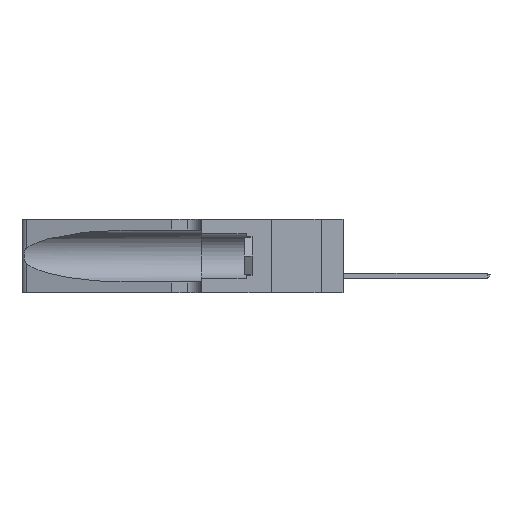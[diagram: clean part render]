
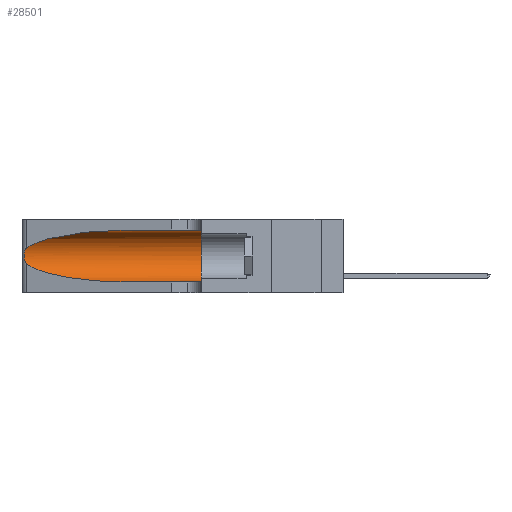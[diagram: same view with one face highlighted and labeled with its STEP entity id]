
A CAD part, left-side view. The second image highlights one B-rep face of the part: STEP entity #28501.
In plain terms, the highlighted cylindrical face has radius 3.308 mm (diameter 6.617 mm), a partial arc.
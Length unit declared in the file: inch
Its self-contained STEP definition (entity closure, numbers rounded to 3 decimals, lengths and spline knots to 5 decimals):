
#901 = VECTOR ( 'NONE', #15719, 39.37008 ) ;
#1679 = DIRECTION ( 'NONE',  ( 0., -1., 0. ) ) ;
#1787 = CARTESIAN_POINT ( 'NONE',  ( 0.1305, 0.72297, 0.31525 ) ) ;
#2654 = CARTESIAN_POINT ( 'NONE',  ( 0.25487, 1.22718, 0.14631 ) ) ;
#3129 = CARTESIAN_POINT ( 'NONE',  ( 0.25487, 1.22718, 0.22369 ) ) ;
#4407 = ORIENTED_EDGE ( 'NONE', *, *, #14760, .F. ) ;
#6469 = EDGE_CURVE ( 'NONE', #27882, #23097, #34751, .T. ) ;
#7777 = CARTESIAN_POINT ( 'NONE',  ( 0.25789, 1.23486, 0.15765 ) ) ;
#8193 = CARTESIAN_POINT ( 'NONE',  ( 0.2373, 1.15595, 0.28018 ) ) ;
#9518 = AXIS2_PLACEMENT_3D ( 'NONE', #21501, #12907, #29490 ) ;
#10396 = DIRECTION ( 'NONE',  ( 0., 0., 1. ) ) ;
#10615 = DIRECTION ( 'NONE',  ( 0., 1., 0. ) ) ;
#10787 = ORIENTED_EDGE ( 'NONE', *, *, #6469, .T. ) ;
#11015 = CARTESIAN_POINT ( 'NONE',  ( 0.1305, 0.72297, 0.31525 ) ) ;
#11675 = CARTESIAN_POINT ( 'NONE',  ( 0.1305, 0.72297, 0.05475 ) ) ;
#12907 = DIRECTION ( 'NONE',  ( 0., -1., 0. ) ) ;
#13051 = EDGE_CURVE ( 'NONE', #18614, #27882, #20097, .T. ) ;
#13065 = EDGE_LOOP ( 'NONE', ( #19049, #10787, #21907, #31096, #4407, #27449 ) ) ;
#13212 = CARTESIAN_POINT ( 'NONE',  ( 0.25639, 1.23186, 0.15144 ) ) ;
#13287 = CARTESIAN_POINT ( 'NONE',  ( 0.25787, 1.23484, 0.2124 ) ) ;
#14752 = CARTESIAN_POINT ( 'NONE',  ( 0.26017, 1.23833, 0.17102 ) ) ;
#14760 = EDGE_CURVE ( 'NONE', #23066, #15373, #33604, .T. ) ;
#15373 = VERTEX_POINT ( 'NONE', #18941 ) ;
#15399 = LINE ( 'NONE', #28543, #28885 ) ;
#15586 = CARTESIAN_POINT ( 'NONE',  ( 0.1305, 1.61858, 0.05475 ) ) ;
#15719 = DIRECTION ( 'NONE',  ( 0., -1., 0. ) ) ;
#16036 = FACE_OUTER_BOUND ( 'NONE', #13065, .T. ) ;
#16269 = CARTESIAN_POINT ( 'NONE',  ( 0.25487, 1.22718, 0.22369 ) ) ;
#17012 = AXIS2_PLACEMENT_3D ( 'NONE', #31837, #10615, #10396 ) ;
#17485 = CARTESIAN_POINT ( 'NONE',  ( 0.25639, 1.23184, 0.21858 ) ) ;
#18572 = CARTESIAN_POINT ( 'NONE',  ( 0.1305, 0.72297, 0.05475 ) ) ;
#18614 = VERTEX_POINT ( 'NONE', #1787 ) ;
#18941 = CARTESIAN_POINT ( 'NONE',  ( 0.1305, 0.35, 0.05475 ) ) ;
#18957 = CARTESIAN_POINT ( 'NONE',  ( 0.25555, 1.22993, 0.14849 ) ) ;
#19049 = ORIENTED_EDGE ( 'NONE', *, *, #13051, .T. ) ;
#19261 = CARTESIAN_POINT ( 'NONE',  ( 0.18966, 0.96281, 0.31525 ) ) ;
#20068 = EDGE_CURVE ( 'NONE', #23097, #29409, #21814, .T. ) ;
#20097 =( BOUNDED_CURVE ( )  B_SPLINE_CURVE ( 3, ( #11015, #19261, #8193, #3129 ),
 .UNSPECIFIED., .F., .F. ) 
 B_SPLINE_CURVE_WITH_KNOTS ( ( 4, 4 ),
 ( 1.5708, 2.84003 ),
 .UNSPECIFIED. ) 
 CURVE ( )  GEOMETRIC_REPRESENTATION_ITEM ( )  RATIONAL_B_SPLINE_CURVE ( ( 1., 0.87, 0.87, 1. ) ) 
 REPRESENTATION_ITEM ( '' )  );
#21279 = CARTESIAN_POINT ( 'NONE',  ( 0.25854, 1.2359, 0.20912 ) ) ;
#21501 = CARTESIAN_POINT ( 'NONE',  ( 0.1305, 1.61858, 0.185 ) ) ;
#21814 =( BOUNDED_CURVE ( )  B_SPLINE_CURVE ( 3, ( #2654, #29160, #25000, #11675 ),
 .UNSPECIFIED., .F., .F. ) 
 B_SPLINE_CURVE_WITH_KNOTS ( ( 4, 4 ),
 ( 3.44316, 4.71239 ),
 .UNSPECIFIED. ) 
 CURVE ( )  GEOMETRIC_REPRESENTATION_ITEM ( )  RATIONAL_B_SPLINE_CURVE ( ( 1., 0.87, 0.87, 1. ) ) 
 REPRESENTATION_ITEM ( '' )  );
#21907 = ORIENTED_EDGE ( 'NONE', *, *, #20068, .T. ) ;
#22245 = EDGE_CURVE ( 'NONE', #29409, #15373, #26633, .T. ) ;
#22837 = CARTESIAN_POINT ( 'NONE',  ( 0.26075, 1.23896, 0.178 ) ) ;
#23066 = VERTEX_POINT ( 'NONE', #32313 ) ;
#23097 = VERTEX_POINT ( 'NONE', #24535 ) ;
#24397 = CARTESIAN_POINT ( 'NONE',  ( 0.25487, 1.22718, 0.14631 ) ) ;
#24535 = CARTESIAN_POINT ( 'NONE',  ( 0.25487, 1.22718, 0.14631 ) ) ;
#25000 = CARTESIAN_POINT ( 'NONE',  ( 0.18966, 0.96281, 0.05475 ) ) ;
#26152 = CARTESIAN_POINT ( 'NONE',  ( 0.26018, 1.23835, 0.19895 ) ) ;
#26425 = EDGE_CURVE ( 'NONE', #18614, #23066, #15399, .T. ) ;
#26633 = LINE ( 'NONE', #15586, #901 ) ;
#27449 = ORIENTED_EDGE ( 'NONE', *, *, #26425, .F. ) ;
#27882 = VERTEX_POINT ( 'NONE', #29416 ) ;
#28501 = ADVANCED_FACE ( 'NONE', ( #16036 ), #33329, .F. ) ;
#28543 = CARTESIAN_POINT ( 'NONE',  ( 0.1305, 1.61858, 0.31525 ) ) ;
#28885 = VECTOR ( 'NONE', #1679, 39.37008 ) ;
#29160 = CARTESIAN_POINT ( 'NONE',  ( 0.2373, 1.15595, 0.08982 ) ) ;
#29409 = VERTEX_POINT ( 'NONE', #18572 ) ;
#29416 = CARTESIAN_POINT ( 'NONE',  ( 0.25487, 1.22718, 0.22369 ) ) ;
#29490 = DIRECTION ( 'NONE',  ( 0., 0., -1. ) ) ;
#31096 = ORIENTED_EDGE ( 'NONE', *, *, #22245, .T. ) ;
#31837 = CARTESIAN_POINT ( 'NONE',  ( 0.1305, 0.35, 0.185 ) ) ;
#32271 = CARTESIAN_POINT ( 'NONE',  ( 0.26075, 1.23896, 0.19203 ) ) ;
#32313 = CARTESIAN_POINT ( 'NONE',  ( 0.1305, 0.35, 0.31525 ) ) ;
#32456 = CARTESIAN_POINT ( 'NONE',  ( 0.25856, 1.23593, 0.16098 ) ) ;
#33329 = CYLINDRICAL_SURFACE ( 'NONE', #9518, 0.13025 ) ;
#33604 = CIRCLE ( 'NONE', #17012, 0.13025 ) ;
#33669 = CARTESIAN_POINT ( 'NONE',  ( 0.25555, 1.22994, 0.2215 ) ) ;
#34751 = B_SPLINE_CURVE_WITH_KNOTS ( 'NONE', 3,
 ( #16269, #33669, #17485, #13287, #21279, #26152, #32271, #22837, #14752, #32456, #7777, #13212, #18957, #24397 ),
 .UNSPECIFIED., .F., .F.,
 ( 4, 2, 2, 2, 2, 2, 4 ),
 ( 0., 0.00027, 0.00053, 0.00107, 0.0016, 0.00187, 0.00214 ),
 .UNSPECIFIED. ) ;
